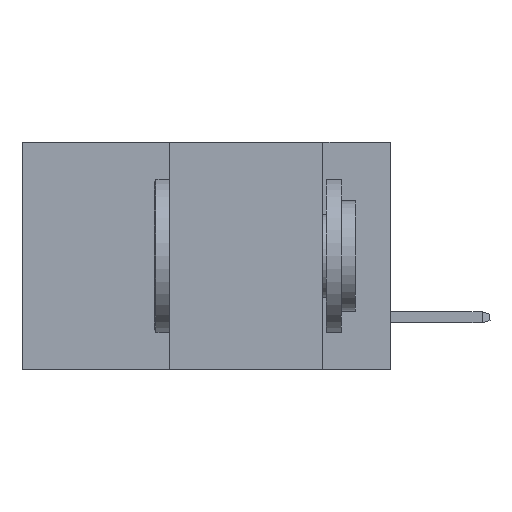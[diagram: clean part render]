
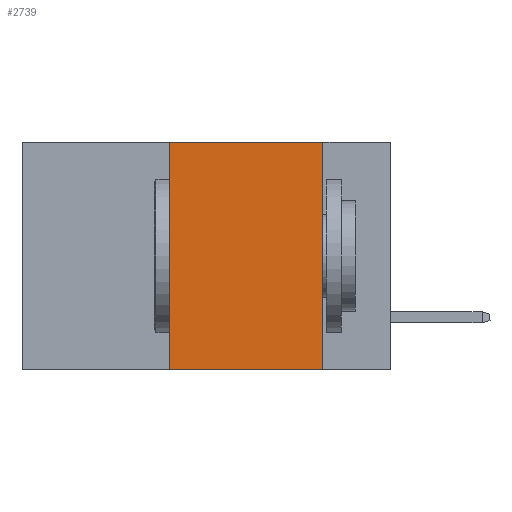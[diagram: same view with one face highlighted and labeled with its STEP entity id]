
A CAD part, left-side view. The second image highlights one B-rep face of the part: STEP entity #2739.
In plain terms, the highlighted planar face has unit normal (-1, 0, 0).
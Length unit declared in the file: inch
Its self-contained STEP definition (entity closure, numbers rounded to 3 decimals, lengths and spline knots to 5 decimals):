
#578 = ORIENTED_EDGE ( 'NONE', *, *, #13746, .F. ) ;
#669 = DIRECTION ( 'NONE',  ( 0., -1., 0. ) ) ;
#874 = CARTESIAN_POINT ( 'NONE',  ( 0., 0.6, 0. ) ) ;
#1001 = VECTOR ( 'NONE', #5701, 39.37008 ) ;
#1709 = VECTOR ( 'NONE', #3615, 39.37008 ) ;
#1971 = ORIENTED_EDGE ( 'NONE', *, *, #3563, .F. ) ;
#2278 = VERTEX_POINT ( 'NONE', #4731 ) ;
#2739 = ADVANCED_FACE ( 'NONE', ( #16916 ), #3468, .F. ) ;
#3397 = DIRECTION ( 'NONE',  ( 0., 0., -1. ) ) ;
#3415 = DIRECTION ( 'NONE',  ( 1., 0., 0. ) ) ;
#3453 = CARTESIAN_POINT ( 'NONE',  ( 0., 0.6, 0. ) ) ;
#3468 = PLANE ( 'NONE',  #12439 ) ;
#3517 = LINE ( 'NONE', #874, #7183 ) ;
#3563 = EDGE_CURVE ( 'NONE', #12902, #13136, #3517, .T. ) ;
#3615 = DIRECTION ( 'NONE',  ( 0., 0., 1. ) ) ;
#4731 = CARTESIAN_POINT ( 'NONE',  ( 0., 0.36, -0.37 ) ) ;
#5215 = ORIENTED_EDGE ( 'NONE', *, *, #15315, .T. ) ;
#5701 = DIRECTION ( 'NONE',  ( 0., 0., -1. ) ) ;
#5950 = ORIENTED_EDGE ( 'NONE', *, *, #14536, .F. ) ;
#7183 = VECTOR ( 'NONE', #669, 39.37008 ) ;
#7872 = DIRECTION ( 'NONE',  ( 0., -1., 0. ) ) ;
#8253 = CARTESIAN_POINT ( 'NONE',  ( 0., 0.11, 0. ) ) ;
#8401 = LINE ( 'NONE', #12176, #1001 ) ;
#8857 = CARTESIAN_POINT ( 'NONE',  ( 0., 0.11, -0.37 ) ) ;
#8998 = VERTEX_POINT ( 'NONE', #8857 ) ;
#11399 = LINE ( 'NONE', #16545, #14275 ) ;
#12176 = CARTESIAN_POINT ( 'NONE',  ( 0., 0.11, 0. ) ) ;
#12423 = LINE ( 'NONE', #15157, #1709 ) ;
#12439 = AXIS2_PLACEMENT_3D ( 'NONE', #3453, #3415, #3397 ) ;
#12902 = VERTEX_POINT ( 'NONE', #16425 ) ;
#13136 = VERTEX_POINT ( 'NONE', #8253 ) ;
#13746 = EDGE_CURVE ( 'NONE', #13136, #8998, #8401, .T. ) ;
#14275 = VECTOR ( 'NONE', #7872, 39.37008 ) ;
#14536 = EDGE_CURVE ( 'NONE', #2278, #12902, #12423, .T. ) ;
#15157 = CARTESIAN_POINT ( 'NONE',  ( 0., 0.36, 0. ) ) ;
#15315 = EDGE_CURVE ( 'NONE', #2278, #8998, #11399, .T. ) ;
#16383 = EDGE_LOOP ( 'NONE', ( #578, #1971, #5950, #5215 ) ) ;
#16425 = CARTESIAN_POINT ( 'NONE',  ( 0., 0.36, 0. ) ) ;
#16545 = CARTESIAN_POINT ( 'NONE',  ( 0., 0.6, -0.37 ) ) ;
#16916 = FACE_OUTER_BOUND ( 'NONE', #16383, .T. ) ;
